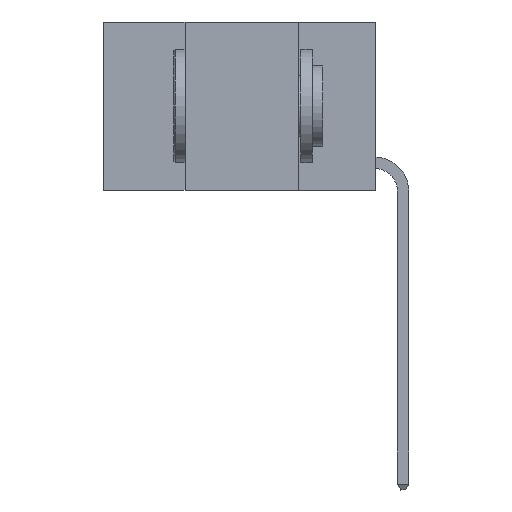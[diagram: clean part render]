
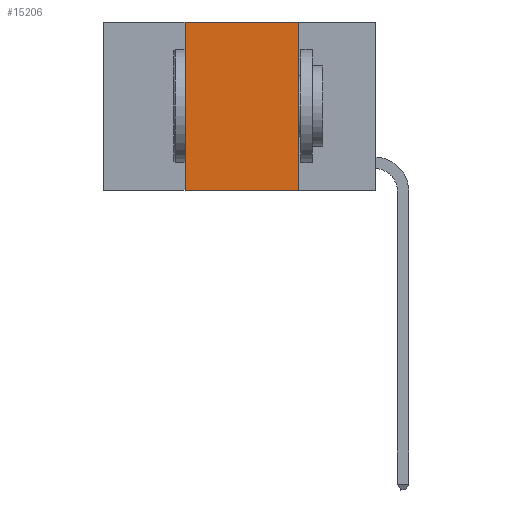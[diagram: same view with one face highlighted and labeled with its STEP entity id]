
A CAD part, left-side view. The second image highlights one B-rep face of the part: STEP entity #15206.
In plain terms, the highlighted planar face has unit normal (-1, 0, 0).
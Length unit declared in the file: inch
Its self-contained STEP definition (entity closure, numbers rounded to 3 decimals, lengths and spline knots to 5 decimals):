
#112 = CARTESIAN_POINT ( 'NONE',  ( 0., 0.42, 0. ) ) ;
#207 = LINE ( 'NONE', #14240, #29030 ) ;
#2155 = DIRECTION ( 'NONE',  ( 1., 0., 0. ) ) ;
#3973 = ORIENTED_EDGE ( 'NONE', *, *, #14673, .F. ) ;
#4723 = PLANE ( 'NONE',  #16359 ) ;
#5765 = EDGE_LOOP ( 'NONE', ( #9231, #3973, #27248, #10118 ) ) ;
#5790 = LINE ( 'NONE', #19396, #12276 ) ;
#6739 = DIRECTION ( 'NONE',  ( 0., -1., 0. ) ) ;
#6928 = EDGE_CURVE ( 'NONE', #28212, #12475, #17945, .T. ) ;
#9231 = ORIENTED_EDGE ( 'NONE', *, *, #23783, .F. ) ;
#10118 = ORIENTED_EDGE ( 'NONE', *, *, #6928, .T. ) ;
#10675 = DIRECTION ( 'NONE',  ( 0., -1., 0. ) ) ;
#11128 = CARTESIAN_POINT ( 'NONE',  ( 0., 0.17, 0. ) ) ;
#12276 = VECTOR ( 'NONE', #14994, 39.37008 ) ;
#12475 = VERTEX_POINT ( 'NONE', #22602 ) ;
#14240 = CARTESIAN_POINT ( 'NONE',  ( 0., 0.42, 0. ) ) ;
#14673 = EDGE_CURVE ( 'NONE', #15561, #18993, #23172, .T. ) ;
#14994 = DIRECTION ( 'NONE',  ( 0., 0., -1. ) ) ;
#15206 = ADVANCED_FACE ( 'NONE', ( #25373 ), #4723, .F. ) ;
#15561 = VERTEX_POINT ( 'NONE', #112 ) ;
#16359 = AXIS2_PLACEMENT_3D ( 'NONE', #18038, #2155, #18339 ) ;
#17494 = CARTESIAN_POINT ( 'NONE',  ( 0., 0.6, -0.37 ) ) ;
#17945 = LINE ( 'NONE', #17494, #22129 ) ;
#18038 = CARTESIAN_POINT ( 'NONE',  ( 0., 0.6, 0. ) ) ;
#18339 = DIRECTION ( 'NONE',  ( 0., 0., -1. ) ) ;
#18993 = VERTEX_POINT ( 'NONE', #11128 ) ;
#19396 = CARTESIAN_POINT ( 'NONE',  ( 0., 0.17, 0. ) ) ;
#19552 = EDGE_CURVE ( 'NONE', #28212, #15561, #207, .T. ) ;
#21915 = VECTOR ( 'NONE', #6739, 39.37008 ) ;
#22129 = VECTOR ( 'NONE', #10675, 39.37008 ) ;
#22602 = CARTESIAN_POINT ( 'NONE',  ( 0., 0.17, -0.37 ) ) ;
#23172 = LINE ( 'NONE', #25413, #21915 ) ;
#23783 = EDGE_CURVE ( 'NONE', #18993, #12475, #5790, .T. ) ;
#25373 = FACE_OUTER_BOUND ( 'NONE', #5765, .T. ) ;
#25413 = CARTESIAN_POINT ( 'NONE',  ( 0., 0.6, 0. ) ) ;
#25696 = DIRECTION ( 'NONE',  ( 0., 0., 1. ) ) ;
#27248 = ORIENTED_EDGE ( 'NONE', *, *, #19552, .F. ) ;
#28212 = VERTEX_POINT ( 'NONE', #28497 ) ;
#28497 = CARTESIAN_POINT ( 'NONE',  ( 0., 0.42, -0.37 ) ) ;
#29030 = VECTOR ( 'NONE', #25696, 39.37008 ) ;
